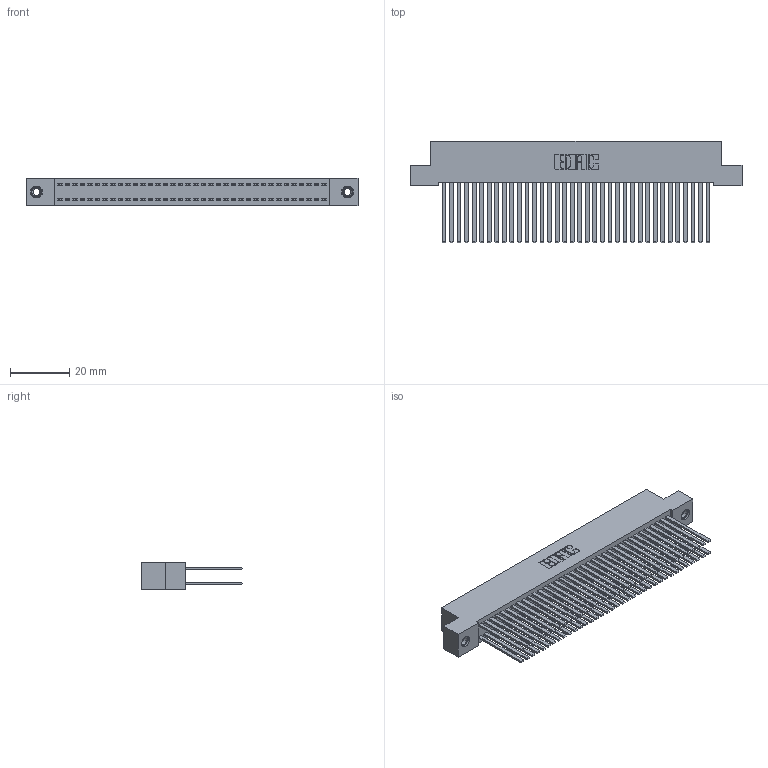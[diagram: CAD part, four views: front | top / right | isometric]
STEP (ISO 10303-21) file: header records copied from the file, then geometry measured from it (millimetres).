
FILE_DESCRIPTION (( 'STEP AP203' ), '1' );
FILE_NAME ('342-072-544-208.STEP', '2018-08-13T10:29:39', ( '' ), ( '' ), 'SwSTEP 2.0', 'SolidWorks 2016', '' );
FILE_SCHEMA (( 'CONFIG_CONTROL_DESIGN' ));
Length unit declared in the file: inch
Products named in the file (4): 342 Part_TI; 345-292-001_345-293-144; 345-250-001_345-250-003-102; 342-072-544-208
Assembly tree (75 placements, depth 2):
  342-072-544-208
    342 Part_TI
    345-292-001_345-293-144  x72
    345-250-001_345-250-003-102  x2
Bounding box: 111.76 x 34.3 x 9.4 mm (x, y, z)
Volume: 11016.8 mm3; surface area: 20590.2 mm2
Topology: 75 solids, 75 shells, 3482 faces, 10299 edges, 6762 vertices
Faces by surface type: plane 2402, cylinder 1064, cone 12, torus 4
Entity records: 24806 total; most frequent: CARTESIAN_POINT 4097, ORIENTED_EDGE 4026, DIRECTION 3539, EDGE_CURVE 2013, VECTOR 1869, LINE 1869, VERTEX_POINT 1336, AXIS2_PLACEMENT_3D 835
